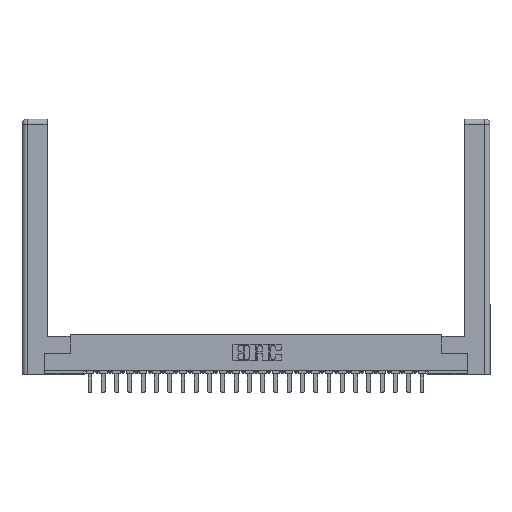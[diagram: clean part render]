
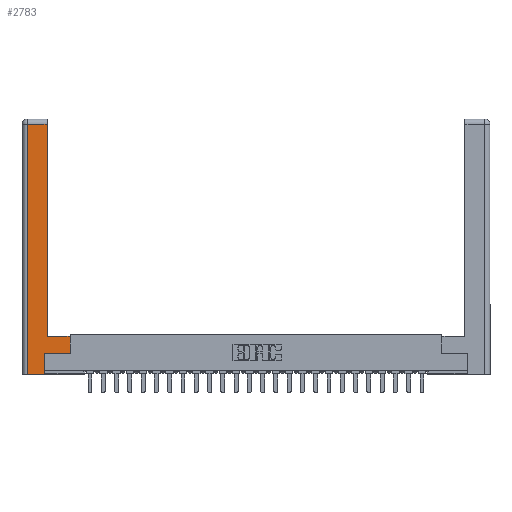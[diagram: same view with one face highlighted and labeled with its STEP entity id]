
A CAD part, top view. The second image highlights one B-rep face of the part: STEP entity #2783.
In plain terms, the highlighted planar face has unit normal (0, 0, 1).
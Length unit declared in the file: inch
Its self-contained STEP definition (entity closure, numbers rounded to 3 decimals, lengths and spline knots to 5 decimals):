
#171 = VERTEX_POINT ( 'NONE', #11392 ) ;
#451 = VECTOR ( 'NONE', #1085, 39.37008 ) ;
#545 = AXIS2_PLACEMENT_3D ( 'NONE', #12318, #27118, #22937 ) ;
#815 = ORIENTED_EDGE ( 'NONE', *, *, #18781, .T. ) ;
#1085 = DIRECTION ( 'NONE',  ( -1., 0., 0. ) ) ;
#1318 = EDGE_CURVE ( 'NONE', #19015, #2084, #4927, .T. ) ;
#1689 = FACE_OUTER_BOUND ( 'NONE', #2169, .T. ) ;
#1955 = CARTESIAN_POINT ( 'NONE',  ( 0.265, 0., 0. ) ) ;
#2031 = CARTESIAN_POINT ( 'NONE',  ( 0.295, 0.45, 0. ) ) ;
#2084 = VERTEX_POINT ( 'NONE', #2031 ) ;
#2169 = EDGE_LOOP ( 'NONE', ( #3728, #22836, #815, #20238, #9203, #26052, #11078, #17241 ) ) ;
#2279 = DIRECTION ( 'NONE',  ( -1., 0., 0. ) ) ;
#2783 = ADVANCED_FACE ( 'NONE', ( #1689 ), #23066, .F. ) ;
#3728 = ORIENTED_EDGE ( 'NONE', *, *, #7674, .T. ) ;
#3778 = DIRECTION ( 'NONE',  ( 1., 0., 0. ) ) ;
#3830 = CARTESIAN_POINT ( 'NONE',  ( 0.295, 3., 0. ) ) ;
#4335 = CARTESIAN_POINT ( 'NONE',  ( 0.295, 2.94, 0. ) ) ;
#4838 = EDGE_CURVE ( 'NONE', #11715, #15186, #20489, .T. ) ;
#4927 = LINE ( 'NONE', #23945, #10774 ) ;
#7424 = EDGE_CURVE ( 'NONE', #19189, #19015, #25805, .T. ) ;
#7674 = EDGE_CURVE ( 'NONE', #2084, #11715, #22982, .T. ) ;
#7681 = VECTOR ( 'NONE', #8112, 39.37008 ) ;
#7700 = CARTESIAN_POINT ( 'NONE',  ( 0.265, 0.245, 0. ) ) ;
#8003 = VECTOR ( 'NONE', #25438, 39.37008 ) ;
#8112 = DIRECTION ( 'NONE',  ( 1., 0., 0. ) ) ;
#8806 = DIRECTION ( 'NONE',  ( 0., -1., 0. ) ) ;
#9203 = ORIENTED_EDGE ( 'NONE', *, *, #12765, .T. ) ;
#10251 = EDGE_CURVE ( 'NONE', #20323, #19189, #16355, .T. ) ;
#10341 = EDGE_CURVE ( 'NONE', #171, #26615, #18729, .T. ) ;
#10774 = VECTOR ( 'NONE', #2279, 39.37008 ) ;
#11078 = ORIENTED_EDGE ( 'NONE', *, *, #7424, .T. ) ;
#11392 = CARTESIAN_POINT ( 'NONE',  ( 0.0615, 0., 0. ) ) ;
#11715 = VERTEX_POINT ( 'NONE', #4335 ) ;
#12318 = CARTESIAN_POINT ( 'NONE',  ( 0., 0., 0. ) ) ;
#12765 = EDGE_CURVE ( 'NONE', #26615, #20323, #16648, .T. ) ;
#13424 = CARTESIAN_POINT ( 'NONE',  ( 0.0615, 2.94, 0. ) ) ;
#13946 = VECTOR ( 'NONE', #24127, 39.37008 ) ;
#14078 = CARTESIAN_POINT ( 'NONE',  ( 0.0615, 2.94, 0. ) ) ;
#15186 = VERTEX_POINT ( 'NONE', #13424 ) ;
#15228 = LINE ( 'NONE', #26129, #18694 ) ;
#15467 = CARTESIAN_POINT ( 'NONE',  ( 0.565, 0.245, 0. ) ) ;
#16355 = LINE ( 'NONE', #16773, #24621 ) ;
#16648 = LINE ( 'NONE', #25298, #8003 ) ;
#16773 = CARTESIAN_POINT ( 'NONE',  ( 0.565, 0.245, 0. ) ) ;
#17241 = ORIENTED_EDGE ( 'NONE', *, *, #1318, .T. ) ;
#18098 = CARTESIAN_POINT ( 'NONE',  ( 0.565, 0.45, 0. ) ) ;
#18694 = VECTOR ( 'NONE', #8806, 39.37008 ) ;
#18729 = LINE ( 'NONE', #1955, #7681 ) ;
#18781 = EDGE_CURVE ( 'NONE', #15186, #171, #15228, .T. ) ;
#18786 = DIRECTION ( 'NONE',  ( 0., 1., 0. ) ) ;
#19015 = VERTEX_POINT ( 'NONE', #26937 ) ;
#19189 = VERTEX_POINT ( 'NONE', #15467 ) ;
#20238 = ORIENTED_EDGE ( 'NONE', *, *, #10341, .T. ) ;
#20323 = VERTEX_POINT ( 'NONE', #7700 ) ;
#20489 = LINE ( 'NONE', #14078, #451 ) ;
#21446 = CARTESIAN_POINT ( 'NONE',  ( 0.265, 0., 0. ) ) ;
#22441 = VECTOR ( 'NONE', #18786, 39.37008 ) ;
#22836 = ORIENTED_EDGE ( 'NONE', *, *, #4838, .T. ) ;
#22937 = DIRECTION ( 'NONE',  ( -1., 0., 0. ) ) ;
#22982 = LINE ( 'NONE', #3830, #22441 ) ;
#23066 = PLANE ( 'NONE',  #545 ) ;
#23945 = CARTESIAN_POINT ( 'NONE',  ( 0.295, 0.45, 0. ) ) ;
#24127 = DIRECTION ( 'NONE',  ( 0., 1., 0. ) ) ;
#24621 = VECTOR ( 'NONE', #3778, 39.37008 ) ;
#25298 = CARTESIAN_POINT ( 'NONE',  ( 0.265, 0.245, 0. ) ) ;
#25438 = DIRECTION ( 'NONE',  ( 0., 1., 0. ) ) ;
#25805 = LINE ( 'NONE', #18098, #13946 ) ;
#26052 = ORIENTED_EDGE ( 'NONE', *, *, #10251, .T. ) ;
#26129 = CARTESIAN_POINT ( 'NONE',  ( 0.0615, 0., 0. ) ) ;
#26615 = VERTEX_POINT ( 'NONE', #21446 ) ;
#26937 = CARTESIAN_POINT ( 'NONE',  ( 0.565, 0.45, 0. ) ) ;
#27118 = DIRECTION ( 'NONE',  ( 0., 0., -1. ) ) ;
